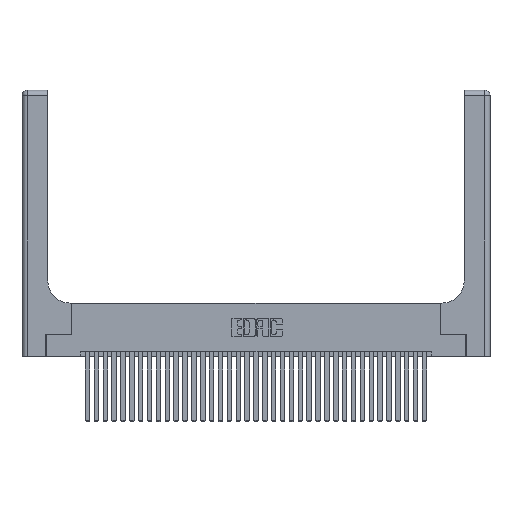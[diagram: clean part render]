
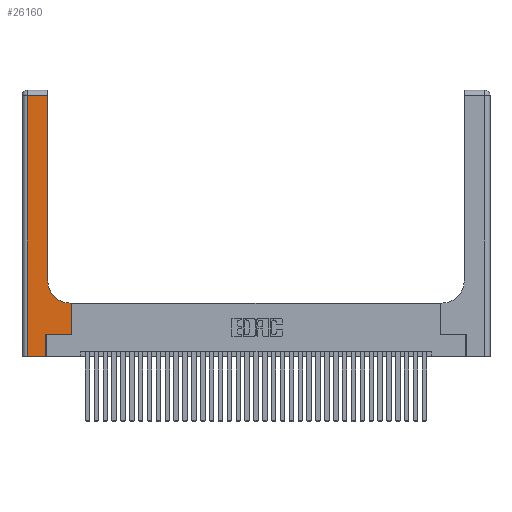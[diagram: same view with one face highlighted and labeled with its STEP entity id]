
A CAD part, top view. The second image highlights one B-rep face of the part: STEP entity #26160.
In plain terms, the highlighted planar face has unit normal (0, 0, 1).
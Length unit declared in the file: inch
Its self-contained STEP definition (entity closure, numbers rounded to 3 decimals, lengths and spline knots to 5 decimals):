
#639 = DIRECTION ( 'NONE',  ( 0., 1., 0. ) ) ;
#683 = VERTEX_POINT ( 'NONE', #13112 ) ;
#807 = CARTESIAN_POINT ( 'NONE',  ( 0.5585, 0.25, 0.37 ) ) ;
#1071 = VERTEX_POINT ( 'NONE', #23034 ) ;
#2731 = VERTEX_POINT ( 'NONE', #25216 ) ;
#2822 = VERTEX_POINT ( 'NONE', #14903 ) ;
#4099 = CARTESIAN_POINT ( 'NONE',  ( 0.5585, 0.25, 0.37 ) ) ;
#4734 = EDGE_CURVE ( 'NONE', #27319, #2822, #26248, .T. ) ;
#5152 = EDGE_CURVE ( 'NONE', #7370, #19958, #13218, .T. ) ;
#5353 = VECTOR ( 'NONE', #32736, 39.37008 ) ;
#5471 = ORIENTED_EDGE ( 'NONE', *, *, #24540, .T. ) ;
#5660 = FACE_OUTER_BOUND ( 'NONE', #7988, .T. ) ;
#6278 = ORIENTED_EDGE ( 'NONE', *, *, #23856, .T. ) ;
#6782 = VECTOR ( 'NONE', #28161, 39.37008 ) ;
#7370 = VERTEX_POINT ( 'NONE', #23582 ) ;
#7988 = EDGE_LOOP ( 'NONE', ( #33904, #5471, #6278, #14654, #12763, #31060, #33918, #22121, #13784 ) ) ;
#8238 = CARTESIAN_POINT ( 'NONE',  ( 0.269, 0.25, 0.37 ) ) ;
#8723 = CARTESIAN_POINT ( 'NONE',  ( 0.2915, 3., 0.37 ) ) ;
#8775 = CARTESIAN_POINT ( 'NONE',  ( 0.269, 0., 0.37 ) ) ;
#8792 = CARTESIAN_POINT ( 'NONE',  ( 0.5415, 0.85, 0.37 ) ) ;
#9730 = EDGE_CURVE ( 'NONE', #2731, #32652, #14250, .T. ) ;
#9910 = AXIS2_PLACEMENT_3D ( 'NONE', #8792, #28232, #11631 ) ;
#11506 = VECTOR ( 'NONE', #31430, 39.37008 ) ;
#11631 = DIRECTION ( 'NONE',  ( 1., 0., 0. ) ) ;
#12325 = VECTOR ( 'NONE', #19353, 39.37008 ) ;
#12763 = ORIENTED_EDGE ( 'NONE', *, *, #31239, .T. ) ;
#13112 = CARTESIAN_POINT ( 'NONE',  ( 0.06, 2.94, 0.37 ) ) ;
#13218 = LINE ( 'NONE', #24778, #12325 ) ;
#13784 = ORIENTED_EDGE ( 'NONE', *, *, #23154, .T. ) ;
#14250 = LINE ( 'NONE', #8723, #6782 ) ;
#14654 = ORIENTED_EDGE ( 'NONE', *, *, #5152, .T. ) ;
#14903 = CARTESIAN_POINT ( 'NONE',  ( 0.5585, 0.6, 0.37 ) ) ;
#15197 = DIRECTION ( 'NONE',  ( -1., 0., 0. ) ) ;
#16065 = DIRECTION ( 'NONE',  ( 0., -1., 0. ) ) ;
#16136 = VECTOR ( 'NONE', #18578, 39.37008 ) ;
#16474 = LINE ( 'NONE', #20164, #22133 ) ;
#16718 = CARTESIAN_POINT ( 'NONE',  ( 0.2915, 2.94, 0.37 ) ) ;
#18578 = DIRECTION ( 'NONE',  ( 1., 0., 0. ) ) ;
#19169 = EDGE_CURVE ( 'NONE', #2822, #1071, #34610, .T. ) ;
#19353 = DIRECTION ( 'NONE',  ( 1., 0., 0. ) ) ;
#19476 = DIRECTION ( 'NONE',  ( -1., 0., 0. ) ) ;
#19913 = VECTOR ( 'NONE', #19476, 39.37008 ) ;
#19958 = VERTEX_POINT ( 'NONE', #8775 ) ;
#20164 = CARTESIAN_POINT ( 'NONE',  ( 0.269, 0., 0.37 ) ) ;
#21051 = LINE ( 'NONE', #32865, #5353 ) ;
#21383 = CARTESIAN_POINT ( 'NONE',  ( 0.269, 0.25, 0.37 ) ) ;
#22121 = ORIENTED_EDGE ( 'NONE', *, *, #19169, .T. ) ;
#22133 = VECTOR ( 'NONE', #639, 39.37008 ) ;
#22256 = CARTESIAN_POINT ( 'NONE',  ( 0.2915, 0.6, 0.37 ) ) ;
#22958 = EDGE_CURVE ( 'NONE', #23961, #27319, #30863, .T. ) ;
#23034 = CARTESIAN_POINT ( 'NONE',  ( 0.5415, 0.6, 0.37 ) ) ;
#23154 = EDGE_CURVE ( 'NONE', #1071, #2731, #34107, .T. ) ;
#23582 = CARTESIAN_POINT ( 'NONE',  ( 0.06, 0., 0.37 ) ) ;
#23856 = EDGE_CURVE ( 'NONE', #683, #7370, #27133, .T. ) ;
#23961 = VERTEX_POINT ( 'NONE', #8238 ) ;
#24540 = EDGE_CURVE ( 'NONE', #32652, #683, #21051, .T. ) ;
#24778 = CARTESIAN_POINT ( 'NONE',  ( 0., 0., 0.37 ) ) ;
#25216 = CARTESIAN_POINT ( 'NONE',  ( 0.2915, 0.85, 0.37 ) ) ;
#26160 = ADVANCED_FACE ( 'NONE', ( #5660 ), #28978, .F. ) ;
#26248 = LINE ( 'NONE', #807, #11506 ) ;
#27133 = LINE ( 'NONE', #32657, #35369 ) ;
#27319 = VERTEX_POINT ( 'NONE', #4099 ) ;
#28161 = DIRECTION ( 'NONE',  ( 0., 1., 0. ) ) ;
#28232 = DIRECTION ( 'NONE',  ( 0., 0., -1. ) ) ;
#28978 = PLANE ( 'NONE',  #32288 ) ;
#30863 = LINE ( 'NONE', #21383, #16136 ) ;
#31060 = ORIENTED_EDGE ( 'NONE', *, *, #22958, .T. ) ;
#31239 = EDGE_CURVE ( 'NONE', #19958, #23961, #16474, .T. ) ;
#31430 = DIRECTION ( 'NONE',  ( 0., 1., 0. ) ) ;
#31767 = DIRECTION ( 'NONE',  ( 0., 0., -1. ) ) ;
#32288 = AXIS2_PLACEMENT_3D ( 'NONE', #34431, #31767, #15197 ) ;
#32652 = VERTEX_POINT ( 'NONE', #16718 ) ;
#32657 = CARTESIAN_POINT ( 'NONE',  ( 0.06, 3., 0.37 ) ) ;
#32736 = DIRECTION ( 'NONE',  ( -1., 0., 0. ) ) ;
#32865 = CARTESIAN_POINT ( 'NONE',  ( 0., 2.94, 0.37 ) ) ;
#33904 = ORIENTED_EDGE ( 'NONE', *, *, #9730, .T. ) ;
#33918 = ORIENTED_EDGE ( 'NONE', *, *, #4734, .T. ) ;
#34107 = CIRCLE ( 'NONE', #9910, 0.25 ) ;
#34431 = CARTESIAN_POINT ( 'NONE',  ( 0., 3., 0.37 ) ) ;
#34610 = LINE ( 'NONE', #22256, #19913 ) ;
#35369 = VECTOR ( 'NONE', #16065, 39.37008 ) ;
